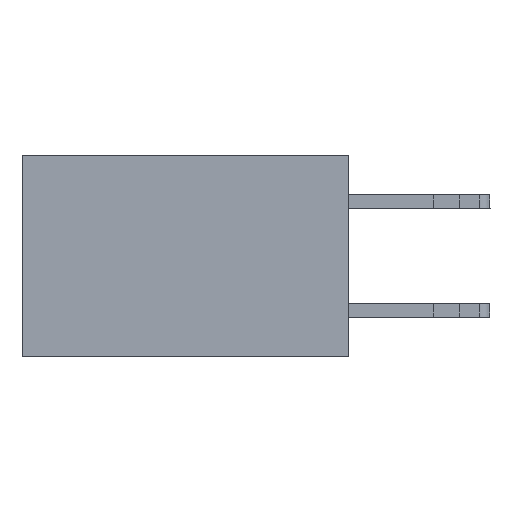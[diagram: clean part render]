
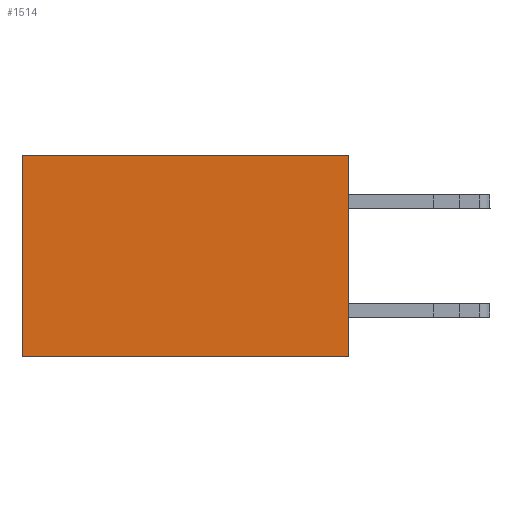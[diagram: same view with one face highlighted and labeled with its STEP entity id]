
A CAD part, left-side view. The second image highlights one B-rep face of the part: STEP entity #1514.
In plain terms, the highlighted planar face has unit normal (-1, 0, 0).
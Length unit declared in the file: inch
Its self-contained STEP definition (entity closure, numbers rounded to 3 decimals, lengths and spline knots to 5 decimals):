
#12 = DIRECTION ( 'NONE',  ( 0., 1., 0. ) ) ;
#798 = CARTESIAN_POINT ( 'NONE',  ( 0.2615, 0.6, 0. ) ) ;
#801 = LINE ( 'NONE', #8086, #12835 ) ;
#832 = EDGE_CURVE ( 'NONE', #13188, #3849, #11467, .T. ) ;
#1204 = LINE ( 'NONE', #4349, #9896 ) ;
#1514 = ADVANCED_FACE ( 'NONE', ( #5665 ), #8897, .F. ) ;
#1532 = DIRECTION ( 'NONE',  ( 1., 0., 0. ) ) ;
#1627 = VECTOR ( 'NONE', #3259, 39.37008 ) ;
#1852 = DIRECTION ( 'NONE',  ( 0., 0., -1. ) ) ;
#2537 = CARTESIAN_POINT ( 'NONE',  ( 0.2615, 0., 0. ) ) ;
#3259 = DIRECTION ( 'NONE',  ( 0., 1., 0. ) ) ;
#3324 = EDGE_LOOP ( 'NONE', ( #13313, #6048, #11517, #9472 ) ) ;
#3849 = VERTEX_POINT ( 'NONE', #10115 ) ;
#3891 = CARTESIAN_POINT ( 'NONE',  ( 0.2615, 0.6, -0.37 ) ) ;
#4240 = AXIS2_PLACEMENT_3D ( 'NONE', #11356, #1532, #7908 ) ;
#4349 = CARTESIAN_POINT ( 'NONE',  ( 0.2615, 0., -0.37 ) ) ;
#4898 = EDGE_CURVE ( 'NONE', #8132, #3849, #1204, .T. ) ;
#5118 = VERTEX_POINT ( 'NONE', #2537 ) ;
#5143 = DIRECTION ( 'NONE',  ( 0., 0., -1. ) ) ;
#5665 = FACE_OUTER_BOUND ( 'NONE', #3324, .T. ) ;
#6048 = ORIENTED_EDGE ( 'NONE', *, *, #4898, .F. ) ;
#7488 = EDGE_CURVE ( 'NONE', #5118, #8132, #801, .T. ) ;
#7582 = CARTESIAN_POINT ( 'NONE',  ( 0.2615, 0., 0. ) ) ;
#7908 = DIRECTION ( 'NONE',  ( 0., 0., -1. ) ) ;
#8086 = CARTESIAN_POINT ( 'NONE',  ( 0.2615, 0., -0.37 ) ) ;
#8132 = VERTEX_POINT ( 'NONE', #10730 ) ;
#8897 = PLANE ( 'NONE',  #4240 ) ;
#9472 = ORIENTED_EDGE ( 'NONE', *, *, #12859, .T. ) ;
#9648 = LINE ( 'NONE', #7582, #1627 ) ;
#9896 = VECTOR ( 'NONE', #12, 39.37008 ) ;
#10115 = CARTESIAN_POINT ( 'NONE',  ( 0.2615, 0.6, -0.37 ) ) ;
#10730 = CARTESIAN_POINT ( 'NONE',  ( 0.2615, 0., -0.37 ) ) ;
#11356 = CARTESIAN_POINT ( 'NONE',  ( 0.2615, 0., -0.37 ) ) ;
#11406 = VECTOR ( 'NONE', #1852, 39.37008 ) ;
#11467 = LINE ( 'NONE', #3891, #11406 ) ;
#11517 = ORIENTED_EDGE ( 'NONE', *, *, #7488, .F. ) ;
#12835 = VECTOR ( 'NONE', #5143, 39.37008 ) ;
#12859 = EDGE_CURVE ( 'NONE', #5118, #13188, #9648, .T. ) ;
#13188 = VERTEX_POINT ( 'NONE', #798 ) ;
#13313 = ORIENTED_EDGE ( 'NONE', *, *, #832, .T. ) ;
